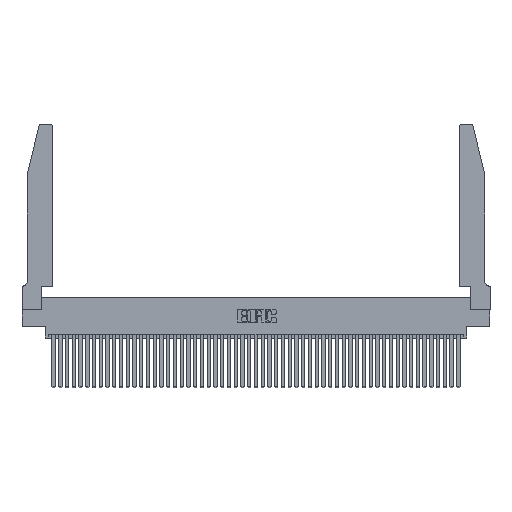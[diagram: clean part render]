
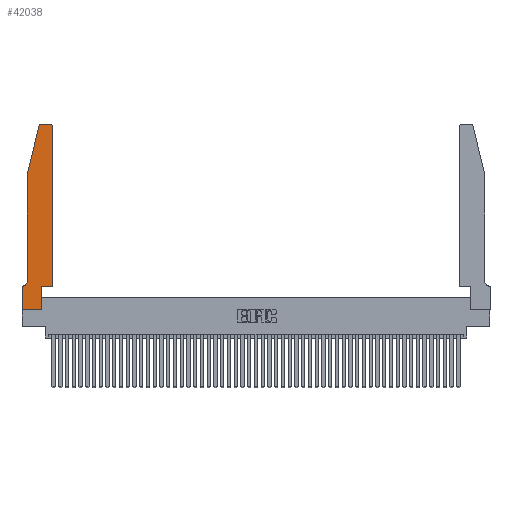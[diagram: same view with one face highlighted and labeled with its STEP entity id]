
A CAD part, top view. The second image highlights one B-rep face of the part: STEP entity #42038.
In plain terms, the highlighted planar face has unit normal (0, 0, 1).
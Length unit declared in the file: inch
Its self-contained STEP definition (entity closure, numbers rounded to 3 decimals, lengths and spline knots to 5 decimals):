
#460 = LINE ( 'NONE', #31269, #31302 ) ;
#1507 = EDGE_CURVE ( 'NONE', #47995, #25907, #30582, .T. ) ;
#1712 = DIRECTION ( 'NONE',  ( -1., 0., 0. ) ) ;
#1721 = DIRECTION ( 'NONE',  ( 1., 0., 0. ) ) ;
#2665 = ORIENTED_EDGE ( 'NONE', *, *, #1507, .T. ) ;
#2752 = FACE_OUTER_BOUND ( 'NONE', #37731, .T. ) ;
#2808 = CARTESIAN_POINT ( 'NONE',  ( 0.4505, 0.35, 0.37 ) ) ;
#3748 = LINE ( 'NONE', #2808, #33412 ) ;
#4047 = LINE ( 'NONE', #45403, #48174 ) ;
#4978 = VERTEX_POINT ( 'NONE', #34186 ) ;
#5197 = VECTOR ( 'NONE', #30108, 39.37008 ) ;
#5622 = CARTESIAN_POINT ( 'NONE',  ( 0.284, 2.72, 0.37 ) ) ;
#5969 = DIRECTION ( 'NONE',  ( 0., 1., 0. ) ) ;
#6139 = CARTESIAN_POINT ( 'NONE',  ( 0.2865, 0.35, 0.37 ) ) ;
#6875 = CARTESIAN_POINT ( 'NONE',  ( 0., 0., 0.37 ) ) ;
#7194 = ORIENTED_EDGE ( 'NONE', *, *, #29997, .T. ) ;
#7294 = CARTESIAN_POINT ( 'NONE',  ( 0.4505, 0.35, 0.37 ) ) ;
#7486 = VERTEX_POINT ( 'NONE', #6875 ) ;
#8540 = ORIENTED_EDGE ( 'NONE', *, *, #20427, .T. ) ;
#8718 = AXIS2_PLACEMENT_3D ( 'NONE', #20992, #29113, #1712 ) ;
#8814 = EDGE_CURVE ( 'NONE', #25907, #15679, #29774, .T. ) ;
#9170 = DIRECTION ( 'NONE',  ( 0., 0., 1. ) ) ;
#9861 = ORIENTED_EDGE ( 'NONE', *, *, #8814, .T. ) ;
#10759 = CARTESIAN_POINT ( 'NONE',  ( 0.0755, 0.35, 0.37 ) ) ;
#11886 = EDGE_CURVE ( 'NONE', #24416, #47995, #3748, .T. ) ;
#11905 = LINE ( 'NONE', #10759, #45195 ) ;
#12115 = DIRECTION ( 'NONE',  ( 0., 0., 1. ) ) ;
#12315 = VERTEX_POINT ( 'NONE', #27152 ) ;
#12364 = VECTOR ( 'NONE', #41644, 39.37008 ) ;
#13039 = DIRECTION ( 'NONE',  ( 1., 0., 0. ) ) ;
#14438 = CARTESIAN_POINT ( 'NONE',  ( 0., 0., 0.37 ) ) ;
#14582 = EDGE_CURVE ( 'NONE', #18291, #4978, #19308, .T. ) ;
#15141 = CARTESIAN_POINT ( 'NONE',  ( 0.4505, 0.35, 0.37 ) ) ;
#15679 = VERTEX_POINT ( 'NONE', #32570 ) ;
#15784 = ORIENTED_EDGE ( 'NONE', *, *, #44273, .T. ) ;
#15822 = EDGE_CURVE ( 'NONE', #12315, #30628, #4047, .T. ) ;
#15965 = ORIENTED_EDGE ( 'NONE', *, *, #36342, .T. ) ;
#17976 = CARTESIAN_POINT ( 'NONE',  ( 0., 0.35, 0.37 ) ) ;
#18291 = VERTEX_POINT ( 'NONE', #31082 ) ;
#19081 = EDGE_CURVE ( 'NONE', #30628, #40462, #44059, .T. ) ;
#19308 = LINE ( 'NONE', #6139, #24715 ) ;
#19467 = DIRECTION ( 'NONE',  ( 1., 0., 0. ) ) ;
#20427 = EDGE_CURVE ( 'NONE', #4978, #24416, #30594, .T. ) ;
#20992 = CARTESIAN_POINT ( 'NONE',  ( 0.0055, 0.42, 0.37 ) ) ;
#21010 = ORIENTED_EDGE ( 'NONE', *, *, #14582, .T. ) ;
#21163 = DIRECTION ( 'NONE',  ( 0., 0., 1. ) ) ;
#22049 = DIRECTION ( 'NONE',  ( -0.239, -0.971, 0. ) ) ;
#24266 = PLANE ( 'NONE',  #29378 ) ;
#24416 = VERTEX_POINT ( 'NONE', #15141 ) ;
#24715 = VECTOR ( 'NONE', #5969, 39.37008 ) ;
#25572 = EDGE_CURVE ( 'NONE', #7486, #18291, #460, .T. ) ;
#25610 = ORIENTED_EDGE ( 'NONE', *, *, #19081, .T. ) ;
#25681 = ORIENTED_EDGE ( 'NONE', *, *, #25572, .T. ) ;
#25907 = VERTEX_POINT ( 'NONE', #40587 ) ;
#27152 = CARTESIAN_POINT ( 'NONE',  ( 0.25487, 2.72718, 0.37 ) ) ;
#27435 = ORIENTED_EDGE ( 'NONE', *, *, #40246, .T. ) ;
#28742 = CARTESIAN_POINT ( 'NONE',  ( 0.4205, 2.72, 0.37 ) ) ;
#29113 = DIRECTION ( 'NONE',  ( 0., 0., -1. ) ) ;
#29287 = LINE ( 'NONE', #14438, #12364 ) ;
#29378 = AXIS2_PLACEMENT_3D ( 'NONE', #31353, #12115, #43391 ) ;
#29774 = LINE ( 'NONE', #44147, #47885 ) ;
#29997 = EDGE_CURVE ( 'NONE', #15679, #12315, #43006, .T. ) ;
#30108 = DIRECTION ( 'NONE',  ( 1., 0., 0. ) ) ;
#30582 = CIRCLE ( 'NONE', #32705, 0.03 ) ;
#30594 = LINE ( 'NONE', #7294, #5197 ) ;
#30628 = VERTEX_POINT ( 'NONE', #40581 ) ;
#30705 = DIRECTION ( 'NONE',  ( 0., -1., 0. ) ) ;
#31082 = CARTESIAN_POINT ( 'NONE',  ( 0.2865, 0., 0.37 ) ) ;
#31269 = CARTESIAN_POINT ( 'NONE',  ( 0., 0., 0.37 ) ) ;
#31302 = VECTOR ( 'NONE', #19467, 39.37008 ) ;
#31353 = CARTESIAN_POINT ( 'NONE',  ( 0., 0.35, 0.37 ) ) ;
#31850 = CARTESIAN_POINT ( 'NONE',  ( 0.0755, 0.42, 0.37 ) ) ;
#32303 = DIRECTION ( 'NONE',  ( -1., 0., 0. ) ) ;
#32564 = CARTESIAN_POINT ( 'NONE',  ( 0.4505, 2.72, 0.37 ) ) ;
#32570 = CARTESIAN_POINT ( 'NONE',  ( 0.284, 2.75, 0.37 ) ) ;
#32705 = AXIS2_PLACEMENT_3D ( 'NONE', #28742, #9170, #13039 ) ;
#33056 = ORIENTED_EDGE ( 'NONE', *, *, #15822, .T. ) ;
#33412 = VECTOR ( 'NONE', #48622, 39.37008 ) ;
#34186 = CARTESIAN_POINT ( 'NONE',  ( 0.2865, 0.35, 0.37 ) ) ;
#35175 = ORIENTED_EDGE ( 'NONE', *, *, #11886, .T. ) ;
#36173 = AXIS2_PLACEMENT_3D ( 'NONE', #5622, #21163, #1721 ) ;
#36342 = EDGE_CURVE ( 'NONE', #46914, #7486, #29287, .T. ) ;
#37731 = EDGE_LOOP ( 'NONE', ( #9861, #7194, #33056, #25610, #15784, #27435, #15965, #25681, #21010, #8540, #35175, #2665 ) ) ;
#40246 = EDGE_CURVE ( 'NONE', #43894, #46914, #11905, .T. ) ;
#40462 = VERTEX_POINT ( 'NONE', #31850 ) ;
#40581 = CARTESIAN_POINT ( 'NONE',  ( 0.0755, 2., 0.37 ) ) ;
#40587 = CARTESIAN_POINT ( 'NONE',  ( 0.4205, 2.75, 0.37 ) ) ;
#41644 = DIRECTION ( 'NONE',  ( 0., -1., 0. ) ) ;
#42038 = ADVANCED_FACE ( 'NONE', ( #2752 ), #24266, .T. ) ;
#43006 = CIRCLE ( 'NONE', #36173, 0.03 ) ;
#43391 = DIRECTION ( 'NONE',  ( 1., 0., 0. ) ) ;
#43894 = VERTEX_POINT ( 'NONE', #44737 ) ;
#44059 = LINE ( 'NONE', #46103, #48867 ) ;
#44147 = CARTESIAN_POINT ( 'NONE',  ( 0.2605, 2.75, 0.37 ) ) ;
#44273 = EDGE_CURVE ( 'NONE', #40462, #43894, #47028, .T. ) ;
#44737 = CARTESIAN_POINT ( 'NONE',  ( 0.0055, 0.35, 0.37 ) ) ;
#45195 = VECTOR ( 'NONE', #45896, 39.37008 ) ;
#45403 = CARTESIAN_POINT ( 'NONE',  ( 0.0755, 2., 0.37 ) ) ;
#45896 = DIRECTION ( 'NONE',  ( -1., 0., 0. ) ) ;
#46103 = CARTESIAN_POINT ( 'NONE',  ( 0.0755, 2., 0.37 ) ) ;
#46914 = VERTEX_POINT ( 'NONE', #17976 ) ;
#47028 = CIRCLE ( 'NONE', #8718, 0.07 ) ;
#47885 = VECTOR ( 'NONE', #32303, 39.37008 ) ;
#47995 = VERTEX_POINT ( 'NONE', #32564 ) ;
#48174 = VECTOR ( 'NONE', #22049, 39.37008 ) ;
#48622 = DIRECTION ( 'NONE',  ( 0., 1., 0. ) ) ;
#48867 = VECTOR ( 'NONE', #30705, 39.37008 ) ;
